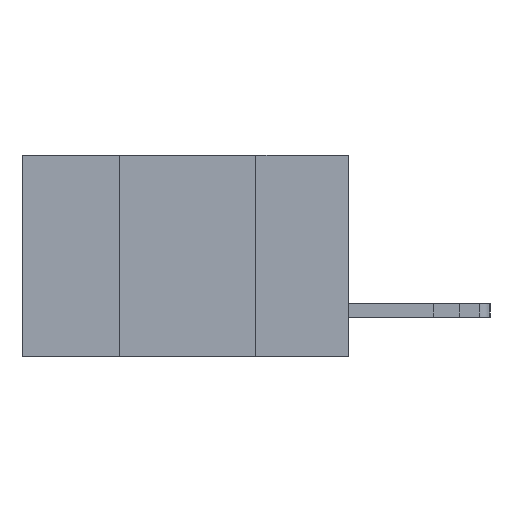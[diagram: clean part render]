
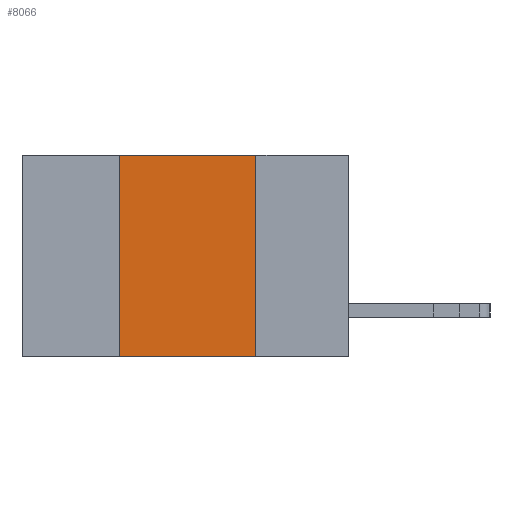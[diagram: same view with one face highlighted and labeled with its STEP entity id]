
A CAD part, left-side view. The second image highlights one B-rep face of the part: STEP entity #8066.
In plain terms, the highlighted planar face has unit normal (-1, 0, 0).
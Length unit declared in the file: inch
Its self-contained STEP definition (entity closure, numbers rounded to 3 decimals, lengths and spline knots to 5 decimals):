
#345 = DIRECTION ( 'NONE',  ( 0., -1., 0. ) ) ;
#507 = FACE_OUTER_BOUND ( 'NONE', #15610, .T. ) ;
#865 = LINE ( 'NONE', #4175, #20708 ) ;
#1398 = LINE ( 'NONE', #18800, #10937 ) ;
#3186 = ORIENTED_EDGE ( 'NONE', *, *, #20435, .F. ) ;
#4175 = CARTESIAN_POINT ( 'NONE',  ( 0., 0.6, -0.37 ) ) ;
#5800 = CARTESIAN_POINT ( 'NONE',  ( 0., 0.6, 0. ) ) ;
#5973 = DIRECTION ( 'NONE',  ( 0., -1., 0. ) ) ;
#6410 = EDGE_CURVE ( 'NONE', #6434, #6684, #1398, .T. ) ;
#6434 = VERTEX_POINT ( 'NONE', #11279 ) ;
#6684 = VERTEX_POINT ( 'NONE', #15465 ) ;
#8066 = ADVANCED_FACE ( 'NONE', ( #507 ), #18103, .F. ) ;
#9079 = LINE ( 'NONE', #10538, #22317 ) ;
#10450 = DIRECTION ( 'NONE',  ( 0., 0., -1. ) ) ;
#10538 = CARTESIAN_POINT ( 'NONE',  ( 0., 0.17, 0. ) ) ;
#10744 = CARTESIAN_POINT ( 'NONE',  ( 0., 0.17, 0. ) ) ;
#10937 = VECTOR ( 'NONE', #13124, 39.37008 ) ;
#11279 = CARTESIAN_POINT ( 'NONE',  ( 0., 0.42, -0.37 ) ) ;
#12626 = EDGE_CURVE ( 'NONE', #6684, #13152, #13530, .T. ) ;
#13124 = DIRECTION ( 'NONE',  ( 0., 0., 1. ) ) ;
#13152 = VERTEX_POINT ( 'NONE', #10744 ) ;
#13530 = LINE ( 'NONE', #5800, #18085 ) ;
#14769 = ORIENTED_EDGE ( 'NONE', *, *, #6410, .F. ) ;
#15465 = CARTESIAN_POINT ( 'NONE',  ( 0., 0.42, 0. ) ) ;
#15610 = EDGE_LOOP ( 'NONE', ( #3186, #20752, #14769, #19912 ) ) ;
#17636 = CARTESIAN_POINT ( 'NONE',  ( 0., 0.17, -0.37 ) ) ;
#18085 = VECTOR ( 'NONE', #345, 39.37008 ) ;
#18103 = PLANE ( 'NONE',  #19367 ) ;
#18150 = DIRECTION ( 'NONE',  ( 0., 0., -1. ) ) ;
#18249 = DIRECTION ( 'NONE',  ( 1., 0., 0. ) ) ;
#18800 = CARTESIAN_POINT ( 'NONE',  ( 0., 0.42, 0. ) ) ;
#18860 = CARTESIAN_POINT ( 'NONE',  ( 0., 0.6, 0. ) ) ;
#19367 = AXIS2_PLACEMENT_3D ( 'NONE', #18860, #18249, #18150 ) ;
#19912 = ORIENTED_EDGE ( 'NONE', *, *, #21989, .T. ) ;
#20435 = EDGE_CURVE ( 'NONE', #13152, #22693, #9079, .T. ) ;
#20708 = VECTOR ( 'NONE', #5973, 39.37008 ) ;
#20752 = ORIENTED_EDGE ( 'NONE', *, *, #12626, .F. ) ;
#21989 = EDGE_CURVE ( 'NONE', #6434, #22693, #865, .T. ) ;
#22317 = VECTOR ( 'NONE', #10450, 39.37008 ) ;
#22693 = VERTEX_POINT ( 'NONE', #17636 ) ;
